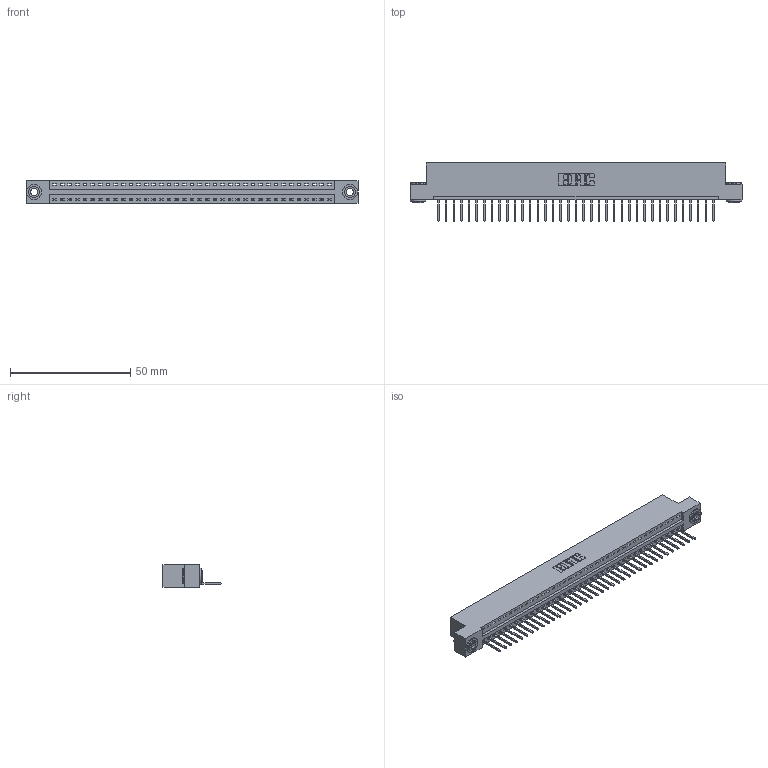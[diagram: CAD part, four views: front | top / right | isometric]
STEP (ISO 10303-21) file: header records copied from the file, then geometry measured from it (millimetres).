
FILE_DESCRIPTION (( 'STEP AP203' ), '1' );
FILE_NAME ('346-037-526-103.STEP', '2018-08-24T03:31:41', ( '' ), ( '' ), 'SwSTEP 2.0', 'SolidWorks 2016', '' );
FILE_SCHEMA (( 'CONFIG_CONTROL_DESIGN' ));
Length unit declared in the file: inch
Products named in the file (4): 346 Part_Flush Mounting Lugs - 0.156 Dia-TH; 345-292-001_345-293-126; 345-250-002_345-250-002-102; 346-037-526-103
Assembly tree (40 placements, depth 2):
  346-037-526-103
    346 Part_Flush Mounting Lugs - 0.156 Dia-TH
    345-292-001_345-293-126  x37
    345-250-002_345-250-002-102  x2
Bounding box: 138.05 x 24.13 x 9.4 mm (x, y, z)
Volume: 13169.8 mm3; surface area: 16589.8 mm2
Topology: 40 solids, 40 shells, 2306 faces, 6917 edges, 4558 vertices
Faces by surface type: plane 1566, cylinder 732, cone 8
Entity records: 24304 total; most frequent: CARTESIAN_POINT 4146, ORIENTED_EDGE 4110, DIRECTION 3695, EDGE_CURVE 2055, LINE 1751, VECTOR 1751, VERTEX_POINT 1366, AXIS2_PLACEMENT_3D 972
